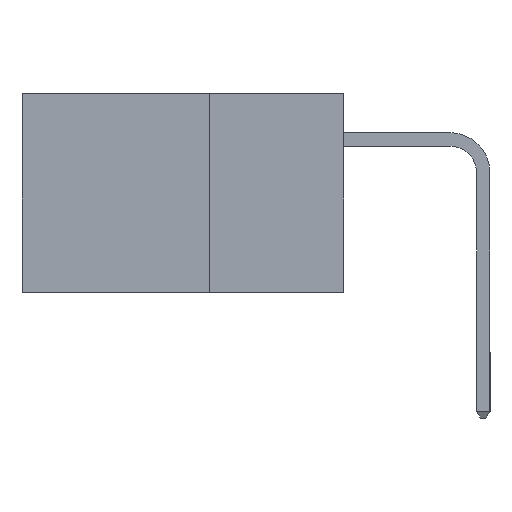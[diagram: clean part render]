
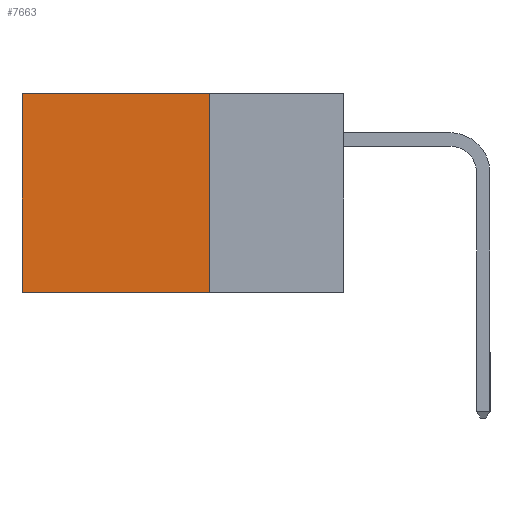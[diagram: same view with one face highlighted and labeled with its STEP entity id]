
A CAD part, left-side view. The second image highlights one B-rep face of the part: STEP entity #7663.
In plain terms, the highlighted planar face has unit normal (-1, 0, 0).
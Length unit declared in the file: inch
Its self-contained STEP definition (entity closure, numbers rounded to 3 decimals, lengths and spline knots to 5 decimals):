
#871 = EDGE_CURVE ( 'NONE', #20638, #9717, #4659, .T. ) ;
#1806 = DIRECTION ( 'NONE',  ( 1., 0., 0. ) ) ;
#3445 = CARTESIAN_POINT ( 'NONE',  ( 0.298, 0.6, -0.37 ) ) ;
#4009 = EDGE_CURVE ( 'NONE', #9717, #22450, #12251, .T. ) ;
#4013 = EDGE_CURVE ( 'NONE', #20638, #14519, #4189, .T. ) ;
#4189 = LINE ( 'NONE', #21069, #18553 ) ;
#4659 = LINE ( 'NONE', #12651, #11285 ) ;
#4716 = CARTESIAN_POINT ( 'NONE',  ( 0.298, 0.25, -0.37 ) ) ;
#5411 = CARTESIAN_POINT ( 'NONE',  ( 0.298, 0.25, 0. ) ) ;
#5797 = DIRECTION ( 'NONE',  ( 0., 0., -1. ) ) ;
#5865 = DIRECTION ( 'NONE',  ( 0., 0., -1. ) ) ;
#5958 = EDGE_LOOP ( 'NONE', ( #7166, #21245, #19760, #16454 ) ) ;
#7166 = ORIENTED_EDGE ( 'NONE', *, *, #14193, .T. ) ;
#7663 = ADVANCED_FACE ( 'NONE', ( #15243 ), #16761, .F. ) ;
#8185 = CARTESIAN_POINT ( 'NONE',  ( 0.298, 0.25, -0.37 ) ) ;
#9717 = VERTEX_POINT ( 'NONE', #4716 ) ;
#10793 = DIRECTION ( 'NONE',  ( 0., 0., -1. ) ) ;
#11285 = VECTOR ( 'NONE', #10793, 39.37008 ) ;
#11671 = VECTOR ( 'NONE', #18965, 39.37008 ) ;
#11909 = DIRECTION ( 'NONE',  ( 0., 1., 0. ) ) ;
#12251 = LINE ( 'NONE', #8185, #11671 ) ;
#12651 = CARTESIAN_POINT ( 'NONE',  ( 0.298, 0.25, 0. ) ) ;
#13527 = AXIS2_PLACEMENT_3D ( 'NONE', #20461, #1806, #5797 ) ;
#14193 = EDGE_CURVE ( 'NONE', #14519, #22450, #21936, .T. ) ;
#14519 = VERTEX_POINT ( 'NONE', #18131 ) ;
#15011 = CARTESIAN_POINT ( 'NONE',  ( 0.298, 0.6, 0. ) ) ;
#15243 = FACE_OUTER_BOUND ( 'NONE', #5958, .T. ) ;
#16454 = ORIENTED_EDGE ( 'NONE', *, *, #4013, .T. ) ;
#16761 = PLANE ( 'NONE',  #13527 ) ;
#18131 = CARTESIAN_POINT ( 'NONE',  ( 0.298, 0.6, 0. ) ) ;
#18553 = VECTOR ( 'NONE', #11909, 39.37008 ) ;
#18965 = DIRECTION ( 'NONE',  ( 0., 1., 0. ) ) ;
#19315 = VECTOR ( 'NONE', #5865, 39.37008 ) ;
#19760 = ORIENTED_EDGE ( 'NONE', *, *, #871, .F. ) ;
#20461 = CARTESIAN_POINT ( 'NONE',  ( 0.298, 0.25, 0. ) ) ;
#20638 = VERTEX_POINT ( 'NONE', #5411 ) ;
#21069 = CARTESIAN_POINT ( 'NONE',  ( 0.298, 0.25, 0. ) ) ;
#21245 = ORIENTED_EDGE ( 'NONE', *, *, #4009, .F. ) ;
#21936 = LINE ( 'NONE', #15011, #19315 ) ;
#22450 = VERTEX_POINT ( 'NONE', #3445 ) ;
